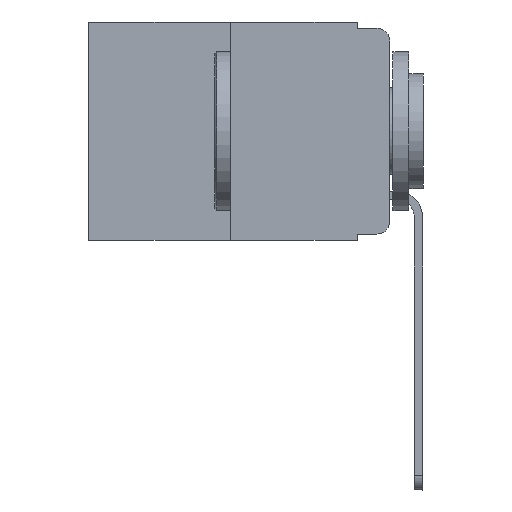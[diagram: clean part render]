
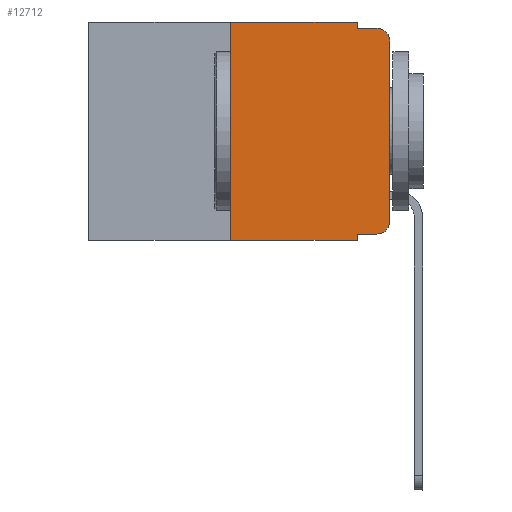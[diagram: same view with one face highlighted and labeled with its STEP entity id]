
A CAD part, left-side view. The second image highlights one B-rep face of the part: STEP entity #12712.
In plain terms, the highlighted planar face has unit normal (-1, 0, 0).
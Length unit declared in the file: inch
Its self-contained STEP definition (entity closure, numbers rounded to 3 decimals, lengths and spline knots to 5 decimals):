
#205 = DIRECTION ( 'NONE',  ( 0., -1., 0. ) ) ;
#234 = CARTESIAN_POINT ( 'NONE',  ( 0., 0., -0.03 ) ) ;
#550 = EDGE_CURVE ( 'NONE', #8265, #13356, #18506, .T. ) ;
#588 = LINE ( 'NONE', #10372, #10043 ) ;
#615 = VERTEX_POINT ( 'NONE', #19032 ) ;
#697 = CIRCLE ( 'NONE', #13605, 0.02 ) ;
#719 = CARTESIAN_POINT ( 'NONE',  ( 0., 0.02, -0.01 ) ) ;
#770 = AXIS2_PLACEMENT_3D ( 'NONE', #1092, #15567, #9388 ) ;
#854 = VERTEX_POINT ( 'NONE', #11759 ) ;
#1092 = CARTESIAN_POINT ( 'NONE',  ( 0., 0.02, -0.313 ) ) ;
#1102 = ORIENTED_EDGE ( 'NONE', *, *, #20086, .T. ) ;
#1425 = AXIS2_PLACEMENT_3D ( 'NONE', #15230, #5323, #2146 ) ;
#1617 = ORIENTED_EDGE ( 'NONE', *, *, #12210, .F. ) ;
#1787 = CARTESIAN_POINT ( 'NONE',  ( 0., 0.051, 0. ) ) ;
#2146 = DIRECTION ( 'NONE',  ( 0., 0., -1. ) ) ;
#2234 = DIRECTION ( 'NONE',  ( 0., 0., -1. ) ) ;
#2534 = CARTESIAN_POINT ( 'NONE',  ( 0., 0., -0.313 ) ) ;
#2631 = ORIENTED_EDGE ( 'NONE', *, *, #550, .T. ) ;
#2871 = EDGE_CURVE ( 'NONE', #854, #20702, #6544, .T. ) ;
#4697 = VECTOR ( 'NONE', #2234, 39.37008 ) ;
#4739 = LINE ( 'NONE', #4851, #8178 ) ;
#4851 = CARTESIAN_POINT ( 'NONE',  ( 0., 0.473, 0. ) ) ;
#5323 = DIRECTION ( 'NONE',  ( 1., 0., 0. ) ) ;
#5652 = ORIENTED_EDGE ( 'NONE', *, *, #11834, .T. ) ;
#5715 = VERTEX_POINT ( 'NONE', #20163 ) ;
#5798 = DIRECTION ( 'NONE',  ( 0., -1., 0. ) ) ;
#5859 = EDGE_CURVE ( 'NONE', #10098, #7247, #10980, .T. ) ;
#6138 = CARTESIAN_POINT ( 'NONE',  ( 0., 0.051, -0.01 ) ) ;
#6544 = LINE ( 'NONE', #13037, #19156 ) ;
#6644 = ORIENTED_EDGE ( 'NONE', *, *, #5859, .T. ) ;
#6987 = EDGE_LOOP ( 'NONE', ( #6644, #13493, #1617, #7899, #14413, #16260, #5652, #17577, #2631, #1102 ) ) ;
#7011 = FACE_OUTER_BOUND ( 'NONE', #6987, .T. ) ;
#7247 = VERTEX_POINT ( 'NONE', #234 ) ;
#7899 = ORIENTED_EDGE ( 'NONE', *, *, #17855, .F. ) ;
#7919 = EDGE_CURVE ( 'NONE', #8265, #5715, #11684, .T. ) ;
#8178 = VECTOR ( 'NONE', #14646, 39.37008 ) ;
#8265 = VERTEX_POINT ( 'NONE', #18272 ) ;
#8864 = CARTESIAN_POINT ( 'NONE',  ( 0., 0., 0. ) ) ;
#9043 = VECTOR ( 'NONE', #9072, 39.37008 ) ;
#9072 = DIRECTION ( 'NONE',  ( 0., 0., 1. ) ) ;
#9388 = DIRECTION ( 'NONE',  ( 0., 0., -1. ) ) ;
#10043 = VECTOR ( 'NONE', #5798, 39.37008 ) ;
#10098 = VERTEX_POINT ( 'NONE', #2534 ) ;
#10372 = CARTESIAN_POINT ( 'NONE',  ( 0., 0.473, -0.343 ) ) ;
#10980 = LINE ( 'NONE', #8864, #9043 ) ;
#11243 = VECTOR ( 'NONE', #11826, 39.37008 ) ;
#11460 = VERTEX_POINT ( 'NONE', #719 ) ;
#11684 = LINE ( 'NONE', #16816, #4697 ) ;
#11759 = CARTESIAN_POINT ( 'NONE',  ( 0., 0.25, -0.343 ) ) ;
#11826 = DIRECTION ( 'NONE',  ( 0., -1., 0. ) ) ;
#11834 = EDGE_CURVE ( 'NONE', #854, #5715, #588, .T. ) ;
#12210 = EDGE_CURVE ( 'NONE', #20580, #11460, #13547, .T. ) ;
#12712 = ADVANCED_FACE ( 'NONE', ( #7011 ), #13624, .F. ) ;
#13037 = CARTESIAN_POINT ( 'NONE',  ( 0., 0.25, 0. ) ) ;
#13249 = CARTESIAN_POINT ( 'NONE',  ( 0., 0.25, 0. ) ) ;
#13356 = VERTEX_POINT ( 'NONE', #15055 ) ;
#13493 = ORIENTED_EDGE ( 'NONE', *, *, #18018, .T. ) ;
#13547 = LINE ( 'NONE', #16750, #11243 ) ;
#13605 = AXIS2_PLACEMENT_3D ( 'NONE', #16683, #18811, #20202 ) ;
#13624 = PLANE ( 'NONE',  #1425 ) ;
#14378 = CIRCLE ( 'NONE', #770, 0.02 ) ;
#14413 = ORIENTED_EDGE ( 'NONE', *, *, #18337, .F. ) ;
#14646 = DIRECTION ( 'NONE',  ( 0., -1., 0. ) ) ;
#14670 = DIRECTION ( 'NONE',  ( 0., 0., -1. ) ) ;
#14756 = VECTOR ( 'NONE', #205, 39.37008 ) ;
#15055 = CARTESIAN_POINT ( 'NONE',  ( 0., 0.02, -0.333 ) ) ;
#15230 = CARTESIAN_POINT ( 'NONE',  ( 0., 0.473, 0. ) ) ;
#15567 = DIRECTION ( 'NONE',  ( -1., 0., 0. ) ) ;
#16260 = ORIENTED_EDGE ( 'NONE', *, *, #2871, .F. ) ;
#16375 = CARTESIAN_POINT ( 'NONE',  ( 0., 0.051, -0.333 ) ) ;
#16683 = CARTESIAN_POINT ( 'NONE',  ( 0., 0.02, -0.03 ) ) ;
#16750 = CARTESIAN_POINT ( 'NONE',  ( 0., 0.051, -0.01 ) ) ;
#16816 = CARTESIAN_POINT ( 'NONE',  ( 0., 0.051, 0. ) ) ;
#17577 = ORIENTED_EDGE ( 'NONE', *, *, #7919, .F. ) ;
#17835 = DIRECTION ( 'NONE',  ( 0., 0., 1. ) ) ;
#17855 = EDGE_CURVE ( 'NONE', #615, #20580, #18273, .T. ) ;
#18018 = EDGE_CURVE ( 'NONE', #7247, #11460, #697, .T. ) ;
#18272 = CARTESIAN_POINT ( 'NONE',  ( 0., 0.051, -0.333 ) ) ;
#18273 = LINE ( 'NONE', #1787, #19441 ) ;
#18337 = EDGE_CURVE ( 'NONE', #20702, #615, #4739, .T. ) ;
#18506 = LINE ( 'NONE', #16375, #14756 ) ;
#18811 = DIRECTION ( 'NONE',  ( -1., 0., 0. ) ) ;
#19032 = CARTESIAN_POINT ( 'NONE',  ( 0., 0.051, 0. ) ) ;
#19156 = VECTOR ( 'NONE', #17835, 39.37008 ) ;
#19441 = VECTOR ( 'NONE', #14670, 39.37008 ) ;
#20086 = EDGE_CURVE ( 'NONE', #13356, #10098, #14378, .T. ) ;
#20163 = CARTESIAN_POINT ( 'NONE',  ( 0., 0.051, -0.343 ) ) ;
#20202 = DIRECTION ( 'NONE',  ( 0., 0., -1. ) ) ;
#20580 = VERTEX_POINT ( 'NONE', #6138 ) ;
#20702 = VERTEX_POINT ( 'NONE', #13249 ) ;
